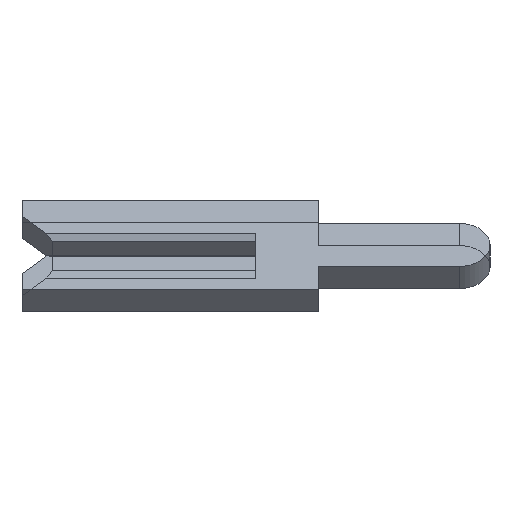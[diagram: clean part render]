
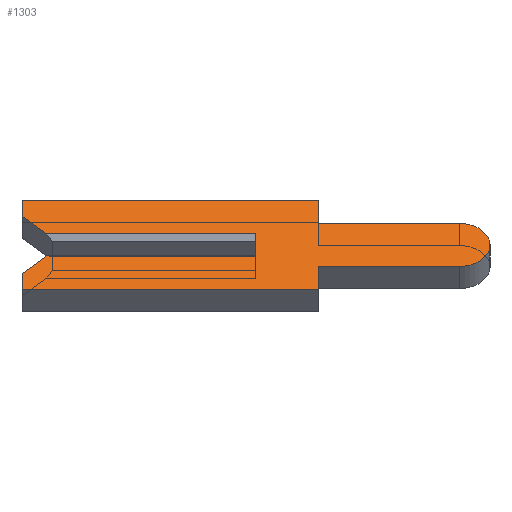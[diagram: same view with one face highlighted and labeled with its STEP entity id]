
A CAD part, left-side view. The second image highlights one B-rep face of the part: STEP entity #1303.
In plain terms, the highlighted face is planar.
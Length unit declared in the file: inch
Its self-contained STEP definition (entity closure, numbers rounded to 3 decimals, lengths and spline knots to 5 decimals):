
#22 = EDGE_CURVE ( 'NONE', #3235, #1855, #2029, .T. ) ;
#67 = VERTEX_POINT ( 'NONE', #1422 ) ;
#88 = VECTOR ( 'NONE', #3260, 39.37008 ) ;
#106 = VERTEX_POINT ( 'NONE', #2195 ) ;
#116 = CIRCLE ( 'NONE', #457, 0.0195 ) ;
#238 = VERTEX_POINT ( 'NONE', #915 ) ;
#246 = CARTESIAN_POINT ( 'NONE',  ( -0.01, 0.15, -0.026 ) ) ;
#271 = DIRECTION ( 'NONE',  ( 0., -1., 0. ) ) ;
#299 = LINE ( 'NONE', #2865, #429 ) ;
#318 = VERTEX_POINT ( 'NONE', #2471 ) ;
#348 = DIRECTION ( 'NONE',  ( 0., 0., -1. ) ) ;
#350 = VERTEX_POINT ( 'NONE', #448 ) ;
#357 = VERTEX_POINT ( 'NONE', #473 ) ;
#381 = ORIENTED_EDGE ( 'NONE', *, *, #22, .F. ) ;
#382 = CARTESIAN_POINT ( 'NONE',  ( -0.01, 0.1305, 0.0065 ) ) ;
#407 = CARTESIAN_POINT ( 'NONE',  ( -0.01, 0.15, -0.04 ) ) ;
#429 = VECTOR ( 'NONE', #271, 39.37008 ) ;
#448 = CARTESIAN_POINT ( 'NONE',  ( -0.01, 0.134, -0.01 ) ) ;
#457 = AXIS2_PLACEMENT_3D ( 'NONE', #1899, #1406, #348 ) ;
#467 = ORIENTED_EDGE ( 'NONE', *, *, #1656, .F. ) ;
#473 = CARTESIAN_POINT ( 'NONE',  ( -0.01, 0.15, -0.026 ) ) ;
#602 = VECTOR ( 'NONE', #2098, 39.37008 ) ;
#609 = DIRECTION ( 'NONE',  ( 0., 0., -1. ) ) ;
#641 = VECTOR ( 'NONE', #1692, 39.37008 ) ;
#651 = DIRECTION ( 'NONE',  ( 0., 1., 0. ) ) ;
#667 = CARTESIAN_POINT ( 'NONE',  ( -0.01, -0.04, -0.0195 ) ) ;
#675 = ORIENTED_EDGE ( 'NONE', *, *, #1872, .F. ) ;
#719 = EDGE_CURVE ( 'NONE', #2595, #357, #1123, .T. ) ;
#765 = ORIENTED_EDGE ( 'NONE', *, *, #1284, .F. ) ;
#792 = CARTESIAN_POINT ( 'NONE',  ( -0.01, -0.04, -0.04 ) ) ;
#812 = ORIENTED_EDGE ( 'NONE', *, *, #2281, .F. ) ;
#856 = CARTESIAN_POINT ( 'NONE',  ( -0.01, 0.15, 0.04 ) ) ;
#903 = LINE ( 'NONE', #2151, #2441 ) ;
#915 = CARTESIAN_POINT ( 'NONE',  ( -0.01, -0.04, 0.04 ) ) ;
#917 = VECTOR ( 'NONE', #1738, 39.37008 ) ;
#931 = EDGE_CURVE ( 'NONE', #2957, #67, #3034, .T. ) ;
#1011 = DIRECTION ( 'NONE',  ( 0., 0., 1. ) ) ;
#1064 = DIRECTION ( 'NONE',  ( 1., 0., 0. ) ) ;
#1080 = VERTEX_POINT ( 'NONE', #2071 ) ;
#1090 = DIRECTION ( 'NONE',  ( 0., 0., -1. ) ) ;
#1123 = LINE ( 'NONE', #246, #3119 ) ;
#1129 = EDGE_LOOP ( 'NONE', ( #1535, #467, #1245, #675, #1132, #1826, #1173, #2624, #3025, #765, #812, #2216, #381, #2590 ) ) ;
#1132 = ORIENTED_EDGE ( 'NONE', *, *, #719, .F. ) ;
#1151 = CARTESIAN_POINT ( 'NONE',  ( -0.01, 0.1305, -0.0065 ) ) ;
#1173 = ORIENTED_EDGE ( 'NONE', *, *, #931, .F. ) ;
#1202 = FACE_OUTER_BOUND ( 'NONE', #1129, .T. ) ;
#1245 = ORIENTED_EDGE ( 'NONE', *, *, #1830, .F. ) ;
#1283 = LINE ( 'NONE', #2679, #2584 ) ;
#1284 = EDGE_CURVE ( 'NONE', #1080, #1578, #299, .T. ) ;
#1303 = ADVANCED_FACE ( 'NONE', ( #1202 ), #2382, .F. ) ;
#1406 = DIRECTION ( 'NONE',  ( 1., 0., 0. ) ) ;
#1418 = EDGE_CURVE ( 'NONE', #2552, #1978, #2668, .T. ) ;
#1422 = CARTESIAN_POINT ( 'NONE',  ( -0.01, -0.04, -0.04 ) ) ;
#1435 = CARTESIAN_POINT ( 'NONE',  ( -0.01, 0.15, 0.026 ) ) ;
#1491 = LINE ( 'NONE', #3244, #917 ) ;
#1535 = ORIENTED_EDGE ( 'NONE', *, *, #1418, .T. ) ;
#1547 = DIRECTION ( 'NONE',  ( 0., 0., -1. ) ) ;
#1578 = VERTEX_POINT ( 'NONE', #2630 ) ;
#1654 = CARTESIAN_POINT ( 'NONE',  ( -0.01, 0., 0.01 ) ) ;
#1656 = EDGE_CURVE ( 'NONE', #318, #1978, #2166, .T. ) ;
#1692 = DIRECTION ( 'NONE',  ( 0., 1., 0. ) ) ;
#1698 = VECTOR ( 'NONE', #1547, 39.37008 ) ;
#1738 = DIRECTION ( 'NONE',  ( 0., -1., 0. ) ) ;
#1826 = ORIENTED_EDGE ( 'NONE', *, *, #2803, .F. ) ;
#1830 = EDGE_CURVE ( 'NONE', #350, #318, #903, .T. ) ;
#1855 = VERTEX_POINT ( 'NONE', #856 ) ;
#1862 = VECTOR ( 'NONE', #2465, 39.37008 ) ;
#1870 = CARTESIAN_POINT ( 'NONE',  ( -0.01, -0.1305, 0. ) ) ;
#1872 = EDGE_CURVE ( 'NONE', #357, #350, #2329, .T. ) ;
#1899 = CARTESIAN_POINT ( 'NONE',  ( -0.01, -0.1305, 0. ) ) ;
#1911 = CARTESIAN_POINT ( 'NONE',  ( -0.01, 0.134, 0.01 ) ) ;
#1978 = VERTEX_POINT ( 'NONE', #1654 ) ;
#2029 = LINE ( 'NONE', #1435, #88 ) ;
#2071 = CARTESIAN_POINT ( 'NONE',  ( -0.01, -0.04, 0.0195 ) ) ;
#2098 = DIRECTION ( 'NONE',  ( 0., -1., 0. ) ) ;
#2151 = CARTESIAN_POINT ( 'NONE',  ( -0.01, -0.1305, -0.01 ) ) ;
#2166 = LINE ( 'NONE', #2181, #2610 ) ;
#2181 = CARTESIAN_POINT ( 'NONE',  ( -0.01, 0., 0.0065 ) ) ;
#2191 = DIRECTION ( 'NONE',  ( 0., -0.707, 0.707 ) ) ;
#2195 = CARTESIAN_POINT ( 'NONE',  ( -0.01, -0.1305, -0.0195 ) ) ;
#2214 = CARTESIAN_POINT ( 'NONE',  ( -0.01, 0.15, -0.04 ) ) ;
#2216 = ORIENTED_EDGE ( 'NONE', *, *, #3243, .F. ) ;
#2281 = EDGE_CURVE ( 'NONE', #238, #1080, #1283, .T. ) ;
#2290 = VECTOR ( 'NONE', #651, 39.37008 ) ;
#2329 = LINE ( 'NONE', #1151, #3024 ) ;
#2347 = EDGE_CURVE ( 'NONE', #1578, #106, #116, .T. ) ;
#2382 = PLANE ( 'NONE',  #2672 ) ;
#2403 = CARTESIAN_POINT ( 'NONE',  ( -0.01, 0.15, 0.01 ) ) ;
#2441 = VECTOR ( 'NONE', #3234, 39.37008 ) ;
#2452 = DIRECTION ( 'NONE',  ( 0., 0., 1. ) ) ;
#2465 = DIRECTION ( 'NONE',  ( 0., 0.707, 0.707 ) ) ;
#2471 = CARTESIAN_POINT ( 'NONE',  ( -0.01, 0., -0.01 ) ) ;
#2512 = CARTESIAN_POINT ( 'NONE',  ( -0.01, -0.04, -0.0195 ) ) ;
#2520 = EDGE_CURVE ( 'NONE', #2552, #3235, #3242, .T. ) ;
#2552 = VERTEX_POINT ( 'NONE', #1911 ) ;
#2584 = VECTOR ( 'NONE', #609, 39.37008 ) ;
#2590 = ORIENTED_EDGE ( 'NONE', *, *, #2520, .F. ) ;
#2595 = VERTEX_POINT ( 'NONE', #407 ) ;
#2610 = VECTOR ( 'NONE', #2452, 39.37008 ) ;
#2624 = ORIENTED_EDGE ( 'NONE', *, *, #2918, .F. ) ;
#2630 = CARTESIAN_POINT ( 'NONE',  ( -0.01, -0.1305, 0.0195 ) ) ;
#2668 = LINE ( 'NONE', #2403, #602 ) ;
#2672 = AXIS2_PLACEMENT_3D ( 'NONE', #1870, #1064, #1090 ) ;
#2679 = CARTESIAN_POINT ( 'NONE',  ( -0.01, -0.04, 0.04 ) ) ;
#2803 = EDGE_CURVE ( 'NONE', #67, #2595, #2975, .T. ) ;
#2865 = CARTESIAN_POINT ( 'NONE',  ( -0.01, -0.04, 0.0195 ) ) ;
#2918 = EDGE_CURVE ( 'NONE', #106, #2957, #3018, .T. ) ;
#2957 = VERTEX_POINT ( 'NONE', #667 ) ;
#2975 = LINE ( 'NONE', #2214, #2290 ) ;
#3018 = LINE ( 'NONE', #2512, #641 ) ;
#3024 = VECTOR ( 'NONE', #2191, 39.37008 ) ;
#3025 = ORIENTED_EDGE ( 'NONE', *, *, #2347, .F. ) ;
#3034 = LINE ( 'NONE', #792, #1698 ) ;
#3037 = CARTESIAN_POINT ( 'NONE',  ( -0.01, 0.15, 0.026 ) ) ;
#3119 = VECTOR ( 'NONE', #1011, 39.37008 ) ;
#3234 = DIRECTION ( 'NONE',  ( 0., -1., 0. ) ) ;
#3235 = VERTEX_POINT ( 'NONE', #3037 ) ;
#3242 = LINE ( 'NONE', #382, #1862 ) ;
#3243 = EDGE_CURVE ( 'NONE', #1855, #238, #1491, .T. ) ;
#3244 = CARTESIAN_POINT ( 'NONE',  ( -0.01, 0.15, 0.04 ) ) ;
#3260 = DIRECTION ( 'NONE',  ( 0., 0., 1. ) ) ;
